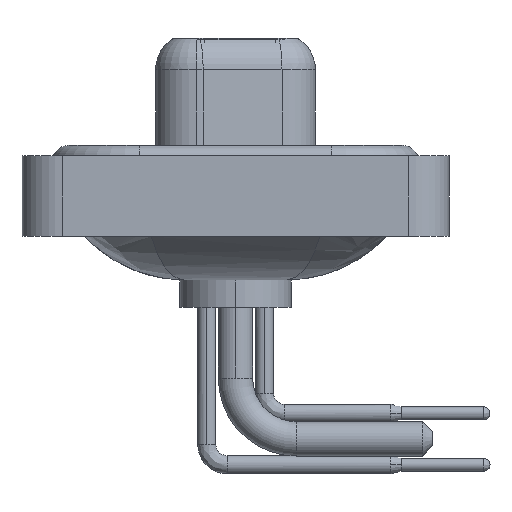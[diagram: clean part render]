
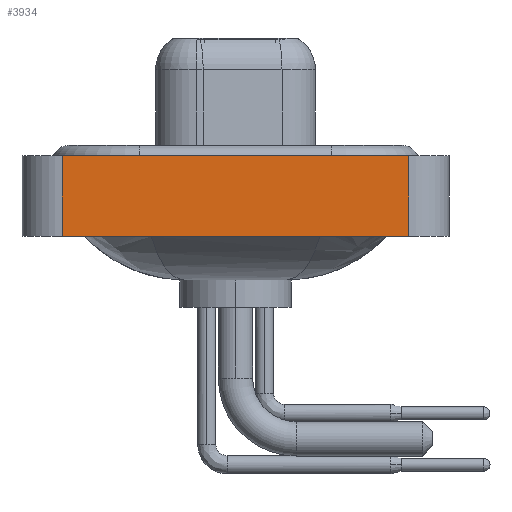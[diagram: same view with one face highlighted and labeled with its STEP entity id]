
A CAD part, left-side view. The second image highlights one B-rep face of the part: STEP entity #3934.
In plain terms, the highlighted planar face has unit normal (-1, 0, 0).
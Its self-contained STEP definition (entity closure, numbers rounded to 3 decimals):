
#290 = LINE ( 'NONE', #7844, #12726 ) ;
#340 = DIRECTION ( 'NONE',  ( 0., 0., 1. ) ) ;
#536 = DIRECTION ( 'NONE',  ( 0., 0., 1. ) ) ;
#833 = VERTEX_POINT ( 'NONE', #1046 ) ;
#1046 = CARTESIAN_POINT ( 'NONE',  ( -7.35, 8.55, 0.4 ) ) ;
#1931 = CARTESIAN_POINT ( 'NONE',  ( -7.35, -8.55, -3.6 ) ) ;
#2027 = VERTEX_POINT ( 'NONE', #13912 ) ;
#2395 = VERTEX_POINT ( 'NONE', #11412 ) ;
#2573 = CARTESIAN_POINT ( 'NONE',  ( -7.35, -8.55, -3.6 ) ) ;
#3227 = AXIS2_PLACEMENT_3D ( 'NONE', #2573, #10122, #340 ) ;
#3934 = ADVANCED_FACE ( 'NONE', ( #23151 ), #6163, .T. ) ;
#4100 = EDGE_CURVE ( 'NONE', #9027, #833, #290, .T. ) ;
#5179 = CARTESIAN_POINT ( 'NONE',  ( -7.35, 8.55, -3.6 ) ) ;
#6163 = PLANE ( 'NONE',  #3227 ) ;
#6735 = EDGE_CURVE ( 'NONE', #833, #2027, #11257, .T. ) ;
#7564 = DIRECTION ( 'NONE',  ( 0., -1., 0. ) ) ;
#7770 = LINE ( 'NONE', #1931, #18837 ) ;
#7844 = CARTESIAN_POINT ( 'NONE',  ( -7.35, 8.55, -3.6 ) ) ;
#8050 = EDGE_LOOP ( 'NONE', ( #12591, #11841, #15656, #17444 ) ) ;
#9027 = VERTEX_POINT ( 'NONE', #5179 ) ;
#10122 = DIRECTION ( 'NONE',  ( -1., 0., 0. ) ) ;
#11002 = CARTESIAN_POINT ( 'NONE',  ( -7.35, -8.55, 0.4 ) ) ;
#11257 = LINE ( 'NONE', #11002, #14065 ) ;
#11412 = CARTESIAN_POINT ( 'NONE',  ( -7.35, -8.55, -3.6 ) ) ;
#11841 = ORIENTED_EDGE ( 'NONE', *, *, #6735, .F. ) ;
#12028 = LINE ( 'NONE', #19614, #16382 ) ;
#12591 = ORIENTED_EDGE ( 'NONE', *, *, #19352, .T. ) ;
#12726 = VECTOR ( 'NONE', #536, 1000. ) ;
#13912 = CARTESIAN_POINT ( 'NONE',  ( -7.35, -8.55, 0.4 ) ) ;
#14065 = VECTOR ( 'NONE', #7564, 1000. ) ;
#15068 = DIRECTION ( 'NONE',  ( 0., 0., 1. ) ) ;
#15656 = ORIENTED_EDGE ( 'NONE', *, *, #4100, .F. ) ;
#16382 = VECTOR ( 'NONE', #23434, 1000. ) ;
#16874 = EDGE_CURVE ( 'NONE', #9027, #2395, #12028, .T. ) ;
#17444 = ORIENTED_EDGE ( 'NONE', *, *, #16874, .T. ) ;
#18837 = VECTOR ( 'NONE', #15068, 1000. ) ;
#19352 = EDGE_CURVE ( 'NONE', #2395, #2027, #7770, .T. ) ;
#19614 = CARTESIAN_POINT ( 'NONE',  ( -7.35, -8.55, -3.6 ) ) ;
#23151 = FACE_OUTER_BOUND ( 'NONE', #8050, .T. ) ;
#23434 = DIRECTION ( 'NONE',  ( 0., -1., 0. ) ) ;
